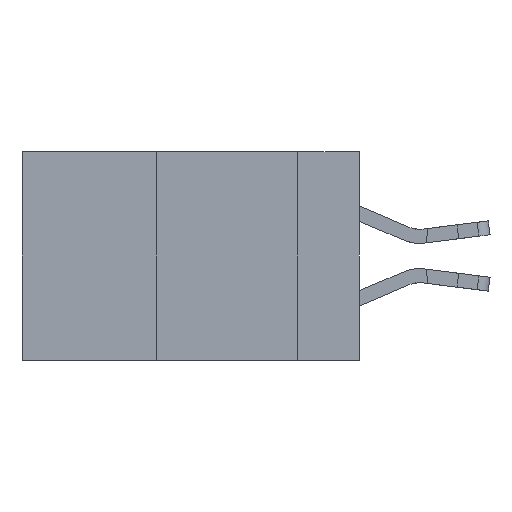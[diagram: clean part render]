
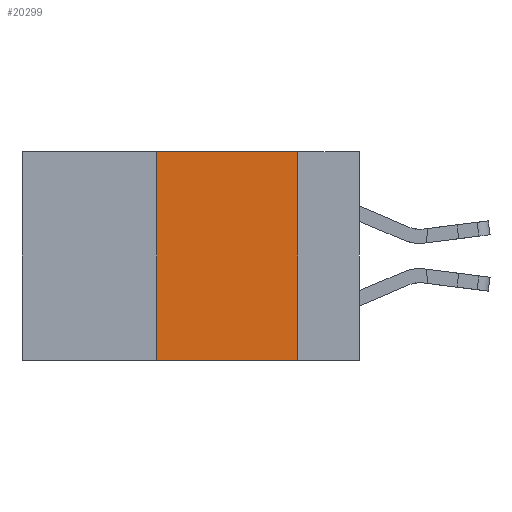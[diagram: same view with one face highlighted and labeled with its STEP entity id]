
A CAD part, left-side view. The second image highlights one B-rep face of the part: STEP entity #20299.
In plain terms, the highlighted planar face has unit normal (-1, 0, 0).
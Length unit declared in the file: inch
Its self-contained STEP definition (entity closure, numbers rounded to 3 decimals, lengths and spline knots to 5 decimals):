
#455 = LINE ( 'NONE', #7881, #12769 ) ;
#888 = PLANE ( 'NONE',  #23149 ) ;
#2707 = EDGE_CURVE ( 'NONE', #4555, #21921, #7677, .T. ) ;
#2815 = LINE ( 'NONE', #14692, #20232 ) ;
#3440 = EDGE_CURVE ( 'NONE', #12247, #4555, #455, .T. ) ;
#4227 = DIRECTION ( 'NONE',  ( 1., 0., 0. ) ) ;
#4555 = VERTEX_POINT ( 'NONE', #10902 ) ;
#4571 = VECTOR ( 'NONE', #17854, 39.37008 ) ;
#5433 = ORIENTED_EDGE ( 'NONE', *, *, #2707, .F. ) ;
#5924 = DIRECTION ( 'NONE',  ( 0., -1., 0. ) ) ;
#7206 = CARTESIAN_POINT ( 'NONE',  ( 0., 0.11, -0.37 ) ) ;
#7677 = LINE ( 'NONE', #16034, #8562 ) ;
#7881 = CARTESIAN_POINT ( 'NONE',  ( 0., 0.6, 0. ) ) ;
#8562 = VECTOR ( 'NONE', #15731, 39.37008 ) ;
#9765 = ORIENTED_EDGE ( 'NONE', *, *, #13516, .T. ) ;
#10532 = ORIENTED_EDGE ( 'NONE', *, *, #17588, .F. ) ;
#10902 = CARTESIAN_POINT ( 'NONE',  ( 0., 0.11, 0. ) ) ;
#11718 = VERTEX_POINT ( 'NONE', #15786 ) ;
#12247 = VERTEX_POINT ( 'NONE', #19645 ) ;
#12286 = ORIENTED_EDGE ( 'NONE', *, *, #3440, .F. ) ;
#12769 = VECTOR ( 'NONE', #5924, 39.37008 ) ;
#13516 = EDGE_CURVE ( 'NONE', #11718, #21921, #17128, .T. ) ;
#13685 = DIRECTION ( 'NONE',  ( 0., 0., -1. ) ) ;
#14692 = CARTESIAN_POINT ( 'NONE',  ( 0., 0.36, 0. ) ) ;
#15731 = DIRECTION ( 'NONE',  ( 0., 0., -1. ) ) ;
#15786 = CARTESIAN_POINT ( 'NONE',  ( 0., 0.36, -0.37 ) ) ;
#16034 = CARTESIAN_POINT ( 'NONE',  ( 0., 0.11, 0. ) ) ;
#17128 = LINE ( 'NONE', #21809, #4571 ) ;
#17588 = EDGE_CURVE ( 'NONE', #11718, #12247, #2815, .T. ) ;
#17854 = DIRECTION ( 'NONE',  ( 0., -1., 0. ) ) ;
#18827 = CARTESIAN_POINT ( 'NONE',  ( 0., 0.6, 0. ) ) ;
#18979 = FACE_OUTER_BOUND ( 'NONE', #20452, .T. ) ;
#19645 = CARTESIAN_POINT ( 'NONE',  ( 0., 0.36, 0. ) ) ;
#20168 = DIRECTION ( 'NONE',  ( 0., 0., 1. ) ) ;
#20232 = VECTOR ( 'NONE', #20168, 39.37008 ) ;
#20299 = ADVANCED_FACE ( 'NONE', ( #18979 ), #888, .F. ) ;
#20452 = EDGE_LOOP ( 'NONE', ( #5433, #12286, #10532, #9765 ) ) ;
#21809 = CARTESIAN_POINT ( 'NONE',  ( 0., 0.6, -0.37 ) ) ;
#21921 = VERTEX_POINT ( 'NONE', #7206 ) ;
#23149 = AXIS2_PLACEMENT_3D ( 'NONE', #18827, #4227, #13685 ) ;
